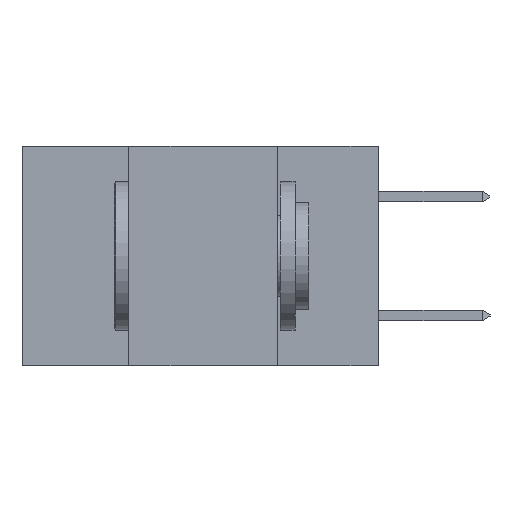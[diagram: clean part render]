
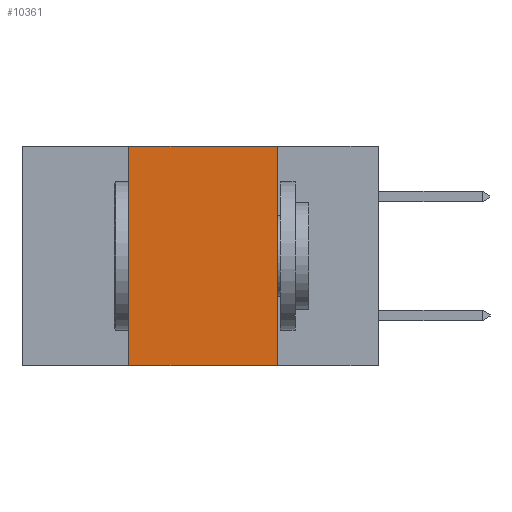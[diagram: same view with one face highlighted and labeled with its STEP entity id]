
A CAD part, left-side view. The second image highlights one B-rep face of the part: STEP entity #10361.
In plain terms, the highlighted planar face has unit normal (-1, 0, 0).
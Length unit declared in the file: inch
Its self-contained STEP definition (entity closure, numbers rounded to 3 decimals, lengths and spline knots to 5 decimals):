
#119 = DIRECTION ( 'NONE',  ( 0., 0., 1. ) ) ;
#652 = EDGE_LOOP ( 'NONE', ( #9339, #5267, #7117, #10421 ) ) ;
#1259 = LINE ( 'NONE', #3526, #3596 ) ;
#1886 = VECTOR ( 'NONE', #119, 39.37008 ) ;
#2924 = CARTESIAN_POINT ( 'NONE',  ( 0., 0.6, 0. ) ) ;
#3143 = DIRECTION ( 'NONE',  ( 0., 0., -1. ) ) ;
#3526 = CARTESIAN_POINT ( 'NONE',  ( 0., 0.6, 0. ) ) ;
#3596 = VECTOR ( 'NONE', #8910, 39.37008 ) ;
#3651 = CARTESIAN_POINT ( 'NONE',  ( 0., 0.42, -0.37 ) ) ;
#4223 = CARTESIAN_POINT ( 'NONE',  ( 0., 0.17, 0. ) ) ;
#4699 = PLANE ( 'NONE',  #6143 ) ;
#5122 = LINE ( 'NONE', #7624, #7322 ) ;
#5174 = EDGE_CURVE ( 'NONE', #7266, #10077, #5122, .T. ) ;
#5267 = ORIENTED_EDGE ( 'NONE', *, *, #10835, .F. ) ;
#5592 = DIRECTION ( 'NONE',  ( 0., 0., -1. ) ) ;
#5790 = VERTEX_POINT ( 'NONE', #9374 ) ;
#6143 = AXIS2_PLACEMENT_3D ( 'NONE', #2924, #10973, #5592 ) ;
#6605 = LINE ( 'NONE', #10532, #8682 ) ;
#7117 = ORIENTED_EDGE ( 'NONE', *, *, #7509, .F. ) ;
#7266 = VERTEX_POINT ( 'NONE', #4223 ) ;
#7322 = VECTOR ( 'NONE', #3143, 39.37008 ) ;
#7509 = EDGE_CURVE ( 'NONE', #5790, #8260, #9004, .T. ) ;
#7624 = CARTESIAN_POINT ( 'NONE',  ( 0., 0.17, -0.37 ) ) ;
#8260 = VERTEX_POINT ( 'NONE', #8851 ) ;
#8682 = VECTOR ( 'NONE', #8695, 39.37008 ) ;
#8695 = DIRECTION ( 'NONE',  ( 0., -1., 0. ) ) ;
#8815 = CARTESIAN_POINT ( 'NONE',  ( 0., 0.17, -0.37 ) ) ;
#8851 = CARTESIAN_POINT ( 'NONE',  ( 0., 0.42, 0. ) ) ;
#8910 = DIRECTION ( 'NONE',  ( 0., -1., 0. ) ) ;
#8952 = FACE_OUTER_BOUND ( 'NONE', #652, .T. ) ;
#9004 = LINE ( 'NONE', #3651, #1886 ) ;
#9339 = ORIENTED_EDGE ( 'NONE', *, *, #5174, .F. ) ;
#9374 = CARTESIAN_POINT ( 'NONE',  ( 0., 0.42, -0.37 ) ) ;
#10007 = EDGE_CURVE ( 'NONE', #5790, #10077, #6605, .T. ) ;
#10077 = VERTEX_POINT ( 'NONE', #8815 ) ;
#10361 = ADVANCED_FACE ( 'NONE', ( #8952 ), #4699, .F. ) ;
#10421 = ORIENTED_EDGE ( 'NONE', *, *, #10007, .T. ) ;
#10532 = CARTESIAN_POINT ( 'NONE',  ( 0., 0.6, -0.37 ) ) ;
#10835 = EDGE_CURVE ( 'NONE', #8260, #7266, #1259, .T. ) ;
#10973 = DIRECTION ( 'NONE',  ( 1., 0., 0. ) ) ;
